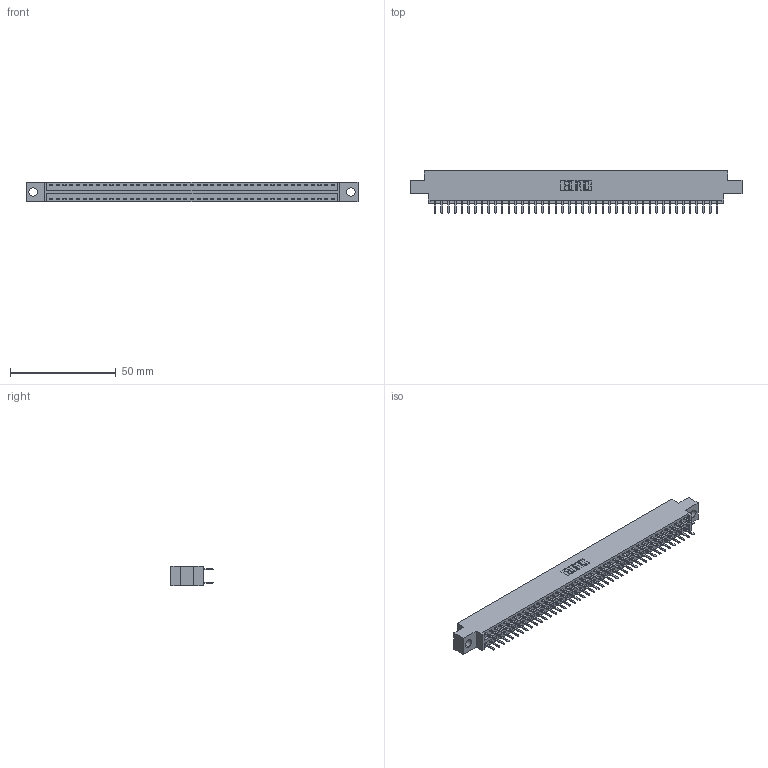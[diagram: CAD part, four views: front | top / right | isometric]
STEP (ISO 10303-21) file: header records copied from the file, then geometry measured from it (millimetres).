
FILE_DESCRIPTION (( 'STEP AP203' ), '1' );
FILE_NAME ('346-086-520-804.STEP', '2022-05-25T21:44:08', ( '' ), ( '' ), 'SwSTEP 2.0', 'SolidWorks 2020', '' );
FILE_SCHEMA (( 'CONFIG_CONTROL_DESIGN' ));
Length unit declared in the file: inch
Products named in the file (3): 346 Part_0.170 Offset - 0.156 Dia-TH; 346-086-520-804; 345-292-001_345-293-120
Assembly tree (87 placements, depth 2):
  346-086-520-804
    346 Part_0.170 Offset - 0.156 Dia-TH
    345-292-001_345-293-120  x86
Bounding box: 157.1 x 20.02 x 9.4 mm (x, y, z)
Volume: 15028.5 mm3; surface area: 20612.3 mm2
Topology: 87 solids, 87 shells, 4956 faces, 14395 edges, 9366 vertices
Faces by surface type: plane 3276, cylinder 1680
Entity records: 28593 total; most frequent: CARTESIAN_POINT 4730, ORIENTED_EDGE 4650, DIRECTION 4205, EDGE_CURVE 2325, LINE 2017, VECTOR 2017, VERTEX_POINT 1546, AXIS2_PLACEMENT_3D 1094
